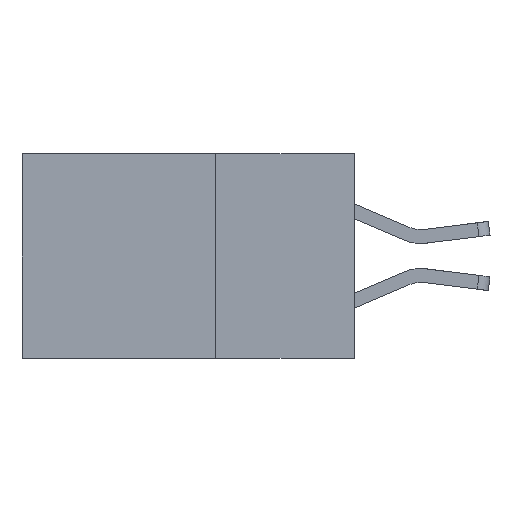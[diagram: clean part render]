
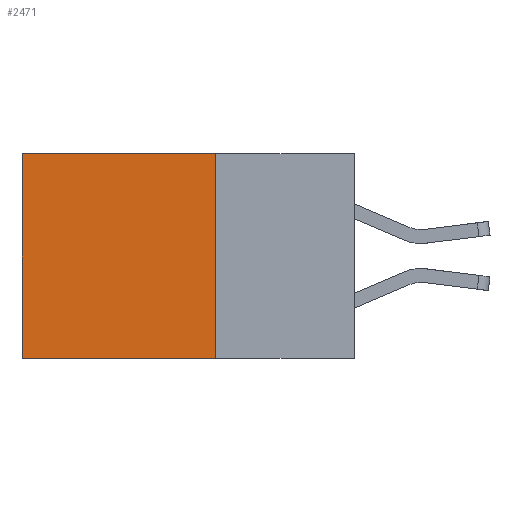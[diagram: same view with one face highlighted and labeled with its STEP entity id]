
A CAD part, left-side view. The second image highlights one B-rep face of the part: STEP entity #2471.
In plain terms, the highlighted planar face has unit normal (-1, 0, 0).
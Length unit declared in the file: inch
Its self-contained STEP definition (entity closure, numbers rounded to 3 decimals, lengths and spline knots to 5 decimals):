
#45 = DIRECTION ( 'NONE',  ( 0., 1., 0. ) ) ;
#117 = VERTEX_POINT ( 'NONE', #9236 ) ;
#322 = AXIS2_PLACEMENT_3D ( 'NONE', #5734, #3565, #1762 ) ;
#589 = ORIENTED_EDGE ( 'NONE', *, *, #7384, .F. ) ;
#702 = EDGE_LOOP ( 'NONE', ( #2743, #7225, #589, #7105 ) ) ;
#1054 = VECTOR ( 'NONE', #3262, 39.37008 ) ;
#1762 = DIRECTION ( 'NONE',  ( 0., 0., -1. ) ) ;
#1936 = DIRECTION ( 'NONE',  ( 0., 0., -1. ) ) ;
#2471 = ADVANCED_FACE ( 'NONE', ( #8158 ), #6446, .F. ) ;
#2510 = CARTESIAN_POINT ( 'NONE',  ( 0.2615, 0.25, -0.37 ) ) ;
#2539 = VECTOR ( 'NONE', #45, 39.37008 ) ;
#2564 = VECTOR ( 'NONE', #1936, 39.37008 ) ;
#2743 = ORIENTED_EDGE ( 'NONE', *, *, #9780, .T. ) ;
#3262 = DIRECTION ( 'NONE',  ( 0., 1., 0. ) ) ;
#3565 = DIRECTION ( 'NONE',  ( 1., 0., 0. ) ) ;
#3944 = VERTEX_POINT ( 'NONE', #2510 ) ;
#4045 = CARTESIAN_POINT ( 'NONE',  ( 0.2615, 0.25, -0.37 ) ) ;
#4901 = LINE ( 'NONE', #4045, #2539 ) ;
#5618 = EDGE_CURVE ( 'NONE', #117, #6122, #5801, .T. ) ;
#5734 = CARTESIAN_POINT ( 'NONE',  ( 0.2615, 0.25, -0.37 ) ) ;
#5801 = LINE ( 'NONE', #7874, #1054 ) ;
#6122 = VERTEX_POINT ( 'NONE', #6661 ) ;
#6296 = VECTOR ( 'NONE', #8918, 39.37008 ) ;
#6446 = PLANE ( 'NONE',  #322 ) ;
#6661 = CARTESIAN_POINT ( 'NONE',  ( 0.2615, 0.6, 0. ) ) ;
#6719 = CARTESIAN_POINT ( 'NONE',  ( 0.2615, 0.6, -0.37 ) ) ;
#6806 = CARTESIAN_POINT ( 'NONE',  ( 0.2615, 0.25, -0.37 ) ) ;
#7105 = ORIENTED_EDGE ( 'NONE', *, *, #5618, .T. ) ;
#7225 = ORIENTED_EDGE ( 'NONE', *, *, #8618, .F. ) ;
#7384 = EDGE_CURVE ( 'NONE', #117, #3944, #9071, .T. ) ;
#7543 = VERTEX_POINT ( 'NONE', #7616 ) ;
#7616 = CARTESIAN_POINT ( 'NONE',  ( 0.2615, 0.6, -0.37 ) ) ;
#7874 = CARTESIAN_POINT ( 'NONE',  ( 0.2615, 0.25, 0. ) ) ;
#8158 = FACE_OUTER_BOUND ( 'NONE', #702, .T. ) ;
#8277 = LINE ( 'NONE', #6719, #2564 ) ;
#8618 = EDGE_CURVE ( 'NONE', #3944, #7543, #4901, .T. ) ;
#8918 = DIRECTION ( 'NONE',  ( 0., 0., -1. ) ) ;
#9071 = LINE ( 'NONE', #6806, #6296 ) ;
#9236 = CARTESIAN_POINT ( 'NONE',  ( 0.2615, 0.25, 0. ) ) ;
#9780 = EDGE_CURVE ( 'NONE', #6122, #7543, #8277, .T. ) ;
